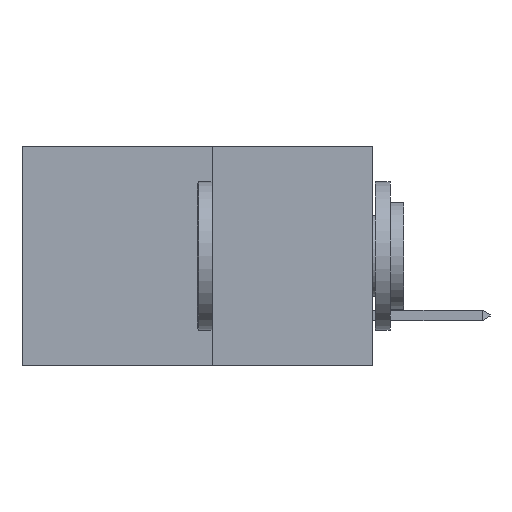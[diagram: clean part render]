
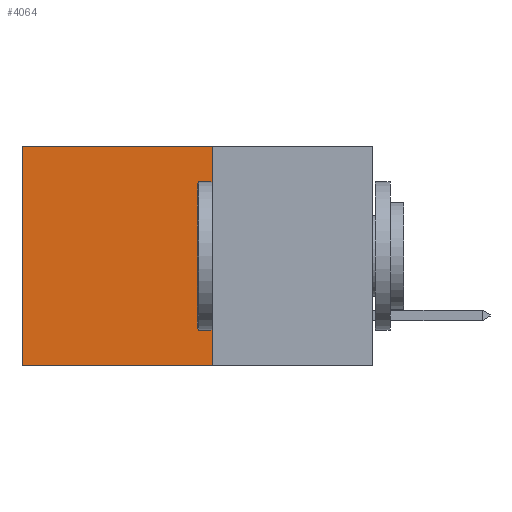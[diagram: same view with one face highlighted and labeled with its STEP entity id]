
A CAD part, left-side view. The second image highlights one B-rep face of the part: STEP entity #4064.
In plain terms, the highlighted planar face has unit normal (-1, 0, 0).
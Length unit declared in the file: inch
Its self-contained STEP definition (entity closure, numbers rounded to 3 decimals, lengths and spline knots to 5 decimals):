
#109 = ORIENTED_EDGE ( 'NONE', *, *, #2625, .F. ) ;
#1313 = VECTOR ( 'NONE', #8732, 39.37008 ) ;
#1844 = VERTEX_POINT ( 'NONE', #8977 ) ;
#2369 = ORIENTED_EDGE ( 'NONE', *, *, #3385, .T. ) ;
#2455 = CARTESIAN_POINT ( 'NONE',  ( 0.277, 0.59, -0.37 ) ) ;
#2625 = EDGE_CURVE ( 'NONE', #6712, #5446, #9354, .T. ) ;
#2754 = DIRECTION ( 'NONE',  ( 0., 0., -1. ) ) ;
#2798 = ORIENTED_EDGE ( 'NONE', *, *, #10916, .T. ) ;
#3252 = DIRECTION ( 'NONE',  ( 1., 0., 0. ) ) ;
#3385 = EDGE_CURVE ( 'NONE', #8946, #5446, #7810, .T. ) ;
#3429 = CARTESIAN_POINT ( 'NONE',  ( 0.277, 0.27, -0.37 ) ) ;
#3857 = CARTESIAN_POINT ( 'NONE',  ( 0.277, 0.27, -0.37 ) ) ;
#3863 = CARTESIAN_POINT ( 'NONE',  ( 0.277, 0.59, 0. ) ) ;
#3872 = AXIS2_PLACEMENT_3D ( 'NONE', #3857, #3252, #2754 ) ;
#4064 = ADVANCED_FACE ( 'NONE', ( #9966 ), #4215, .F. ) ;
#4146 = LINE ( 'NONE', #6847, #10804 ) ;
#4215 = PLANE ( 'NONE',  #3872 ) ;
#4690 = DIRECTION ( 'NONE',  ( 0., 1., 0. ) ) ;
#5446 = VERTEX_POINT ( 'NONE', #2455 ) ;
#5717 = LINE ( 'NONE', #3429, #1313 ) ;
#6712 = VERTEX_POINT ( 'NONE', #6884 ) ;
#6847 = CARTESIAN_POINT ( 'NONE',  ( 0.277, 0.27, 0. ) ) ;
#6884 = CARTESIAN_POINT ( 'NONE',  ( 0.277, 0.27, -0.37 ) ) ;
#6971 = CARTESIAN_POINT ( 'NONE',  ( 0.277, 0.27, -0.37 ) ) ;
#7393 = ORIENTED_EDGE ( 'NONE', *, *, #9747, .F. ) ;
#7781 = DIRECTION ( 'NONE',  ( 0., 1., 0. ) ) ;
#7810 = LINE ( 'NONE', #8833, #9849 ) ;
#8732 = DIRECTION ( 'NONE',  ( 0., 0., -1. ) ) ;
#8833 = CARTESIAN_POINT ( 'NONE',  ( 0.277, 0.59, -0.37 ) ) ;
#8946 = VERTEX_POINT ( 'NONE', #3863 ) ;
#8977 = CARTESIAN_POINT ( 'NONE',  ( 0.277, 0.27, 0. ) ) ;
#9354 = LINE ( 'NONE', #6971, #11271 ) ;
#9747 = EDGE_CURVE ( 'NONE', #1844, #6712, #5717, .T. ) ;
#9849 = VECTOR ( 'NONE', #10756, 39.37008 ) ;
#9966 = FACE_OUTER_BOUND ( 'NONE', #10948, .T. ) ;
#10756 = DIRECTION ( 'NONE',  ( 0., 0., -1. ) ) ;
#10804 = VECTOR ( 'NONE', #7781, 39.37008 ) ;
#10916 = EDGE_CURVE ( 'NONE', #1844, #8946, #4146, .T. ) ;
#10948 = EDGE_LOOP ( 'NONE', ( #2369, #109, #7393, #2798 ) ) ;
#11271 = VECTOR ( 'NONE', #4690, 39.37008 ) ;
